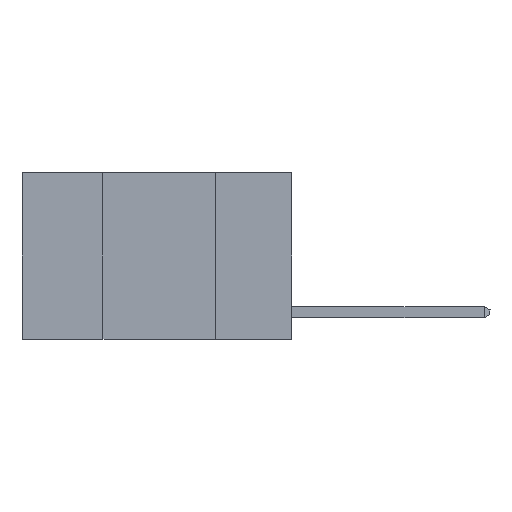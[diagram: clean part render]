
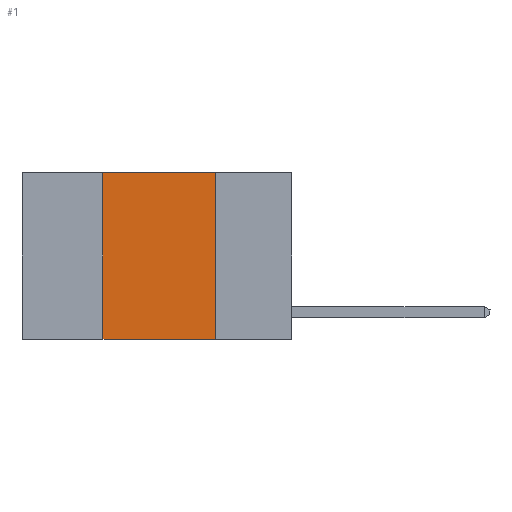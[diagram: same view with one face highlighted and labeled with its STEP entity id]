
A CAD part, left-side view. The second image highlights one B-rep face of the part: STEP entity #1.
In plain terms, the highlighted planar face has unit normal (-1, 0, 0).
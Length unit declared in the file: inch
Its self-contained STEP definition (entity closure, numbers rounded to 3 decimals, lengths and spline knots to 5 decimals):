
#1 = ADVANCED_FACE ( 'NONE', ( #1550 ), #353, .F. ) ;
#353 = PLANE ( 'NONE',  #11119 ) ;
#387 = DIRECTION ( 'NONE',  ( 0., 0., 1. ) ) ;
#702 = EDGE_CURVE ( 'NONE', #11681, #2898, #13120, .T. ) ;
#1131 = DIRECTION ( 'NONE',  ( 0., -1., 0. ) ) ;
#1314 = VECTOR ( 'NONE', #18216, 39.37008 ) ;
#1550 = FACE_OUTER_BOUND ( 'NONE', #4126, .T. ) ;
#1694 = VECTOR ( 'NONE', #387, 39.37008 ) ;
#1862 = ORIENTED_EDGE ( 'NONE', *, *, #16662, .F. ) ;
#1931 = VECTOR ( 'NONE', #1131, 39.37008 ) ;
#2898 = VERTEX_POINT ( 'NONE', #7291 ) ;
#3176 = LINE ( 'NONE', #13046, #8519 ) ;
#3843 = ORIENTED_EDGE ( 'NONE', *, *, #14949, .T. ) ;
#4126 = EDGE_LOOP ( 'NONE', ( #1862, #9799, #13559, #3843 ) ) ;
#4251 = DIRECTION ( 'NONE',  ( 1., 0., 0. ) ) ;
#5049 = VERTEX_POINT ( 'NONE', #15163 ) ;
#6536 = VERTEX_POINT ( 'NONE', #6619 ) ;
#6619 = CARTESIAN_POINT ( 'NONE',  ( 0., 0.17, -0.37 ) ) ;
#7271 = CARTESIAN_POINT ( 'NONE',  ( 0., 0.6, 0. ) ) ;
#7291 = CARTESIAN_POINT ( 'NONE',  ( 0., 0.42, 0. ) ) ;
#8228 = LINE ( 'NONE', #13875, #1931 ) ;
#8519 = VECTOR ( 'NONE', #17061, 39.37008 ) ;
#9799 = ORIENTED_EDGE ( 'NONE', *, *, #14138, .F. ) ;
#11031 = CARTESIAN_POINT ( 'NONE',  ( 0., 0.6, -0.37 ) ) ;
#11119 = AXIS2_PLACEMENT_3D ( 'NONE', #7271, #4251, #11587 ) ;
#11537 = CARTESIAN_POINT ( 'NONE',  ( 0., 0.42, 0. ) ) ;
#11587 = DIRECTION ( 'NONE',  ( 0., 0., -1. ) ) ;
#11681 = VERTEX_POINT ( 'NONE', #11732 ) ;
#11732 = CARTESIAN_POINT ( 'NONE',  ( 0., 0.42, -0.37 ) ) ;
#12621 = LINE ( 'NONE', #11031, #1314 ) ;
#13046 = CARTESIAN_POINT ( 'NONE',  ( 0., 0.17, 0. ) ) ;
#13120 = LINE ( 'NONE', #11537, #1694 ) ;
#13559 = ORIENTED_EDGE ( 'NONE', *, *, #702, .F. ) ;
#13875 = CARTESIAN_POINT ( 'NONE',  ( 0., 0.6, 0. ) ) ;
#14138 = EDGE_CURVE ( 'NONE', #2898, #5049, #8228, .T. ) ;
#14949 = EDGE_CURVE ( 'NONE', #11681, #6536, #12621, .T. ) ;
#15163 = CARTESIAN_POINT ( 'NONE',  ( 0., 0.17, 0. ) ) ;
#16662 = EDGE_CURVE ( 'NONE', #5049, #6536, #3176, .T. ) ;
#17061 = DIRECTION ( 'NONE',  ( 0., 0., -1. ) ) ;
#18216 = DIRECTION ( 'NONE',  ( 0., -1., 0. ) ) ;
